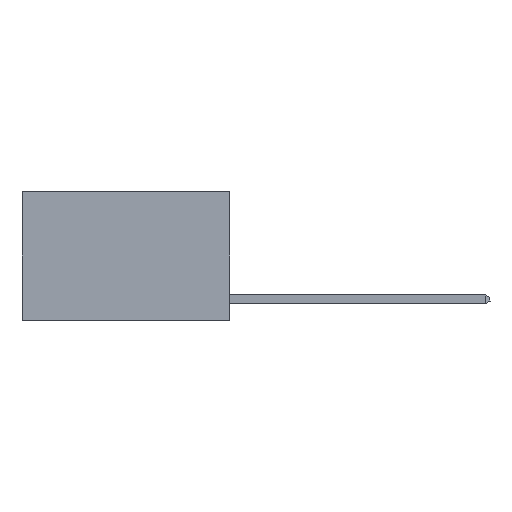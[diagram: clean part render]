
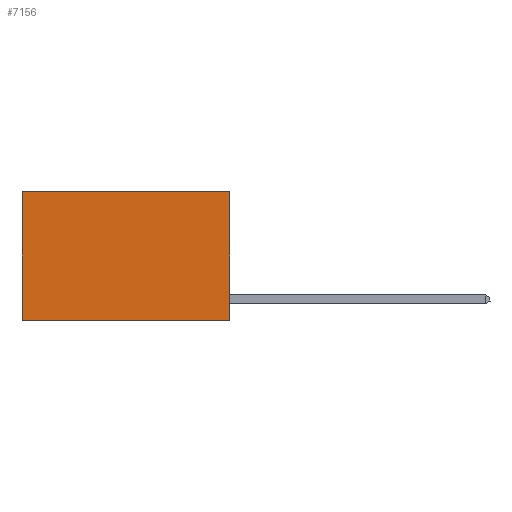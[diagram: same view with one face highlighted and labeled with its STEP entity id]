
A CAD part, left-side view. The second image highlights one B-rep face of the part: STEP entity #7156.
In plain terms, the highlighted planar face has unit normal (-1, 0, 0).
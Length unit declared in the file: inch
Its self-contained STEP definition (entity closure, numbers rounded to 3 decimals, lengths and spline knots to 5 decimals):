
#278 = EDGE_CURVE ( 'NONE', #3313, #3461, #9752, .T. ) ;
#410 = LINE ( 'NONE', #5003, #3129 ) ;
#597 = ORIENTED_EDGE ( 'NONE', *, *, #278, .T. ) ;
#677 = CARTESIAN_POINT ( 'NONE',  ( 0.2625, 0.6, 0. ) ) ;
#1505 = DIRECTION ( 'NONE',  ( 1., 0., 0. ) ) ;
#1854 = DIRECTION ( 'NONE',  ( 0., 0., -1. ) ) ;
#3054 = DIRECTION ( 'NONE',  ( 0., 0., -1. ) ) ;
#3126 = CARTESIAN_POINT ( 'NONE',  ( 0.2625, 0.6, 0. ) ) ;
#3129 = VECTOR ( 'NONE', #1854, 39.37008 ) ;
#3313 = VERTEX_POINT ( 'NONE', #677 ) ;
#3461 = VERTEX_POINT ( 'NONE', #5418 ) ;
#3505 = VERTEX_POINT ( 'NONE', #7893 ) ;
#3648 = DIRECTION ( 'NONE',  ( 0., 1., 0. ) ) ;
#3920 = CARTESIAN_POINT ( 'NONE',  ( 0.2625, 0., 0. ) ) ;
#4241 = ORIENTED_EDGE ( 'NONE', *, *, #7659, .T. ) ;
#4671 = DIRECTION ( 'NONE',  ( 0., 0., -1. ) ) ;
#4773 = FACE_OUTER_BOUND ( 'NONE', #6370, .T. ) ;
#5003 = CARTESIAN_POINT ( 'NONE',  ( 0.2625, 0., 0. ) ) ;
#5418 = CARTESIAN_POINT ( 'NONE',  ( 0.2625, 0.6, -0.37 ) ) ;
#5431 = PLANE ( 'NONE',  #8127 ) ;
#5719 = VECTOR ( 'NONE', #3648, 39.37008 ) ;
#6201 = LINE ( 'NONE', #8408, #5719 ) ;
#6370 = EDGE_LOOP ( 'NONE', ( #597, #6603, #9804, #4241 ) ) ;
#6407 = VECTOR ( 'NONE', #3054, 39.37008 ) ;
#6603 = ORIENTED_EDGE ( 'NONE', *, *, #8947, .F. ) ;
#7156 = ADVANCED_FACE ( 'NONE', ( #4773 ), #5431, .F. ) ;
#7364 = LINE ( 'NONE', #8487, #7864 ) ;
#7659 = EDGE_CURVE ( 'NONE', #7699, #3313, #7364, .T. ) ;
#7699 = VERTEX_POINT ( 'NONE', #3920 ) ;
#7864 = VECTOR ( 'NONE', #10088, 39.37008 ) ;
#7893 = CARTESIAN_POINT ( 'NONE',  ( 0.2625, 0., -0.37 ) ) ;
#8127 = AXIS2_PLACEMENT_3D ( 'NONE', #10141, #1505, #4671 ) ;
#8208 = EDGE_CURVE ( 'NONE', #7699, #3505, #410, .T. ) ;
#8408 = CARTESIAN_POINT ( 'NONE',  ( 0.2625, 0., -0.37 ) ) ;
#8487 = CARTESIAN_POINT ( 'NONE',  ( 0.2625, 0., 0. ) ) ;
#8947 = EDGE_CURVE ( 'NONE', #3505, #3461, #6201, .T. ) ;
#9752 = LINE ( 'NONE', #3126, #6407 ) ;
#9804 = ORIENTED_EDGE ( 'NONE', *, *, #8208, .F. ) ;
#10088 = DIRECTION ( 'NONE',  ( 0., 1., 0. ) ) ;
#10141 = CARTESIAN_POINT ( 'NONE',  ( 0.2625, 0., 0. ) ) ;
